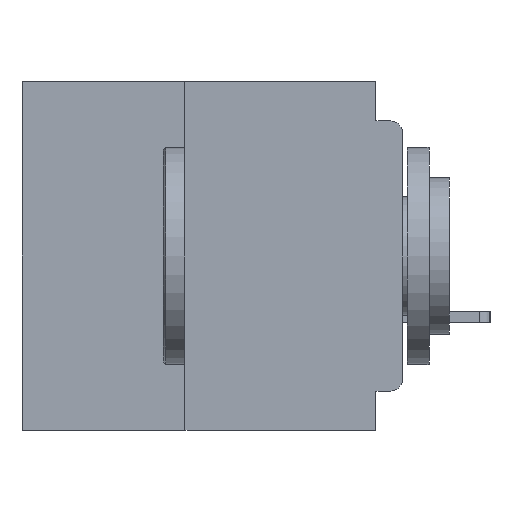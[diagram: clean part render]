
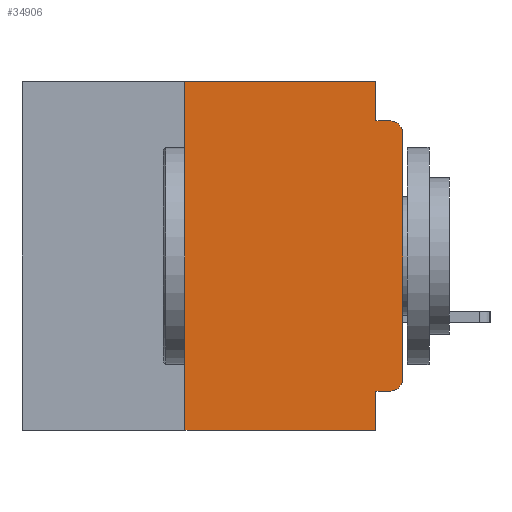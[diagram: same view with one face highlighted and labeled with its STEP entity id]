
A CAD part, left-side view. The second image highlights one B-rep face of the part: STEP entity #34906.
In plain terms, the highlighted planar face has unit normal (-1, 0, 0).
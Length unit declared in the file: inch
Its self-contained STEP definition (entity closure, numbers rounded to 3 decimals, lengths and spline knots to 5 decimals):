
#373 = DIRECTION ( 'NONE',  ( 0., -1., 0. ) ) ;
#462 = CARTESIAN_POINT ( 'NONE',  ( 0., 0., -0.06 ) ) ;
#953 = EDGE_CURVE ( 'NONE', #11437, #25486, #58725, .T. ) ;
#1099 = EDGE_CURVE ( 'NONE', #32701, #32475, #61137, .T. ) ;
#1640 = VECTOR ( 'NONE', #2340, 39.37008 ) ;
#1822 = EDGE_CURVE ( 'NONE', #32701, #12965, #56930, .T. ) ;
#2340 = DIRECTION ( 'NONE',  ( 0., 0., 1. ) ) ;
#2406 = CARTESIAN_POINT ( 'NONE',  ( 0., 0., 0. ) ) ;
#2880 = ORIENTED_EDGE ( 'NONE', *, *, #1822, .F. ) ;
#3015 = CARTESIAN_POINT ( 'NONE',  ( 0., 0.031, -0.4 ) ) ;
#4112 = VECTOR ( 'NONE', #373, 39.37008 ) ;
#5396 = CARTESIAN_POINT ( 'NONE',  ( 0., 0.015, -0.355 ) ) ;
#5739 = CARTESIAN_POINT ( 'NONE',  ( 0., 0.015, -0.06 ) ) ;
#6481 = CARTESIAN_POINT ( 'NONE',  ( 0., 0.25, 0. ) ) ;
#7180 = CARTESIAN_POINT ( 'NONE',  ( 0., 0.437, 0. ) ) ;
#8709 = ORIENTED_EDGE ( 'NONE', *, *, #953, .T. ) ;
#10487 = CIRCLE ( 'NONE', #54897, 0.015 ) ;
#11160 = DIRECTION ( 'NONE',  ( 0., 0., -1. ) ) ;
#11437 = VERTEX_POINT ( 'NONE', #17967 ) ;
#11646 = LINE ( 'NONE', #55209, #38634 ) ;
#11682 = ORIENTED_EDGE ( 'NONE', *, *, #39109, .F. ) ;
#11787 = ORIENTED_EDGE ( 'NONE', *, *, #58823, .F. ) ;
#12354 = VERTEX_POINT ( 'NONE', #67856 ) ;
#12965 = VERTEX_POINT ( 'NONE', #6481 ) ;
#14113 = VERTEX_POINT ( 'NONE', #5396 ) ;
#14119 = VECTOR ( 'NONE', #17174, 39.37008 ) ;
#14875 = EDGE_CURVE ( 'NONE', #12965, #12354, #48651, .T. ) ;
#15000 = CARTESIAN_POINT ( 'NONE',  ( 0., 0.437, 0. ) ) ;
#17174 = DIRECTION ( 'NONE',  ( 0., 0., 1. ) ) ;
#17352 = VERTEX_POINT ( 'NONE', #58790 ) ;
#17586 = CARTESIAN_POINT ( 'NONE',  ( 0., 0., -0.355 ) ) ;
#17967 = CARTESIAN_POINT ( 'NONE',  ( 0., 0., -0.34 ) ) ;
#20053 = VECTOR ( 'NONE', #46953, 39.37008 ) ;
#20403 = PLANE ( 'NONE',  #27753 ) ;
#21796 = VECTOR ( 'NONE', #28850, 39.37008 ) ;
#23650 = ORIENTED_EDGE ( 'NONE', *, *, #29729, .T. ) ;
#23888 = EDGE_CURVE ( 'NONE', #14113, #53511, #45374, .T. ) ;
#24765 = FACE_OUTER_BOUND ( 'NONE', #66228, .T. ) ;
#25486 = VERTEX_POINT ( 'NONE', #462 ) ;
#25836 = DIRECTION ( 'NONE',  ( 0., 0., -1. ) ) ;
#26664 = AXIS2_PLACEMENT_3D ( 'NONE', #5739, #43434, #11160 ) ;
#27753 = AXIS2_PLACEMENT_3D ( 'NONE', #15000, #57922, #25836 ) ;
#28292 = DIRECTION ( 'NONE',  ( 0., -1., 0. ) ) ;
#28850 = DIRECTION ( 'NONE',  ( 0., -1., 0. ) ) ;
#29729 = EDGE_CURVE ( 'NONE', #25486, #45214, #58170, .T. ) ;
#30490 = CARTESIAN_POINT ( 'NONE',  ( 0., 0.031, 0. ) ) ;
#31906 = CARTESIAN_POINT ( 'NONE',  ( 0., 0.015, -0.34 ) ) ;
#32475 = VERTEX_POINT ( 'NONE', #57990 ) ;
#32701 = VERTEX_POINT ( 'NONE', #33370 ) ;
#33370 = CARTESIAN_POINT ( 'NONE',  ( 0., 0.25, -0.4 ) ) ;
#34322 = ORIENTED_EDGE ( 'NONE', *, *, #23888, .F. ) ;
#34906 = ADVANCED_FACE ( 'NONE', ( #24765 ), #20403, .F. ) ;
#37338 = DIRECTION ( 'NONE',  ( 0., 0., -1. ) ) ;
#38634 = VECTOR ( 'NONE', #28292, 39.37008 ) ;
#39109 = EDGE_CURVE ( 'NONE', #17352, #45214, #11646, .T. ) ;
#40455 = LINE ( 'NONE', #3015, #52965 ) ;
#42856 = CARTESIAN_POINT ( 'NONE',  ( 0., 0.015, -0.045 ) ) ;
#42863 = ORIENTED_EDGE ( 'NONE', *, *, #1099, .T. ) ;
#43413 = CARTESIAN_POINT ( 'NONE',  ( 0., 0.437, -0.4 ) ) ;
#43434 = DIRECTION ( 'NONE',  ( -1., 0., 0. ) ) ;
#45214 = VERTEX_POINT ( 'NONE', #42856 ) ;
#45374 = LINE ( 'NONE', #17586, #57897 ) ;
#46050 = DIRECTION ( 'NONE',  ( 0., 0., -1. ) ) ;
#46953 = DIRECTION ( 'NONE',  ( 0., 0., -1. ) ) ;
#48164 = ORIENTED_EDGE ( 'NONE', *, *, #14875, .F. ) ;
#48651 = LINE ( 'NONE', #7180, #21796 ) ;
#52965 = VECTOR ( 'NONE', #46050, 39.37008 ) ;
#53511 = VERTEX_POINT ( 'NONE', #63276 ) ;
#54689 = CARTESIAN_POINT ( 'NONE',  ( 0., 0.25, -0.4 ) ) ;
#54897 = AXIS2_PLACEMENT_3D ( 'NONE', #31906, #69166, #37338 ) ;
#55209 = CARTESIAN_POINT ( 'NONE',  ( 0., 0., -0.045 ) ) ;
#56203 = ORIENTED_EDGE ( 'NONE', *, *, #66600, .F. ) ;
#56930 = LINE ( 'NONE', #54689, #14119 ) ;
#57897 = VECTOR ( 'NONE', #60417, 39.37008 ) ;
#57922 = DIRECTION ( 'NONE',  ( 1., 0., 0. ) ) ;
#57990 = CARTESIAN_POINT ( 'NONE',  ( 0., 0.031, -0.4 ) ) ;
#58170 = CIRCLE ( 'NONE', #26664, 0.015 ) ;
#58618 = ORIENTED_EDGE ( 'NONE', *, *, #62369, .T. ) ;
#58725 = LINE ( 'NONE', #2406, #1640 ) ;
#58790 = CARTESIAN_POINT ( 'NONE',  ( 0., 0.031, -0.045 ) ) ;
#58823 = EDGE_CURVE ( 'NONE', #53511, #32475, #40455, .T. ) ;
#60417 = DIRECTION ( 'NONE',  ( 0., 1., 0. ) ) ;
#61137 = LINE ( 'NONE', #43413, #4112 ) ;
#62369 = EDGE_CURVE ( 'NONE', #14113, #11437, #10487, .T. ) ;
#62738 = LINE ( 'NONE', #30490, #20053 ) ;
#63276 = CARTESIAN_POINT ( 'NONE',  ( 0., 0.031, -0.355 ) ) ;
#66228 = EDGE_LOOP ( 'NONE', ( #8709, #23650, #11682, #56203, #48164, #2880, #42863, #11787, #34322, #58618 ) ) ;
#66600 = EDGE_CURVE ( 'NONE', #12354, #17352, #62738, .T. ) ;
#67856 = CARTESIAN_POINT ( 'NONE',  ( 0., 0.031, 0. ) ) ;
#69166 = DIRECTION ( 'NONE',  ( -1., 0., 0. ) ) ;
